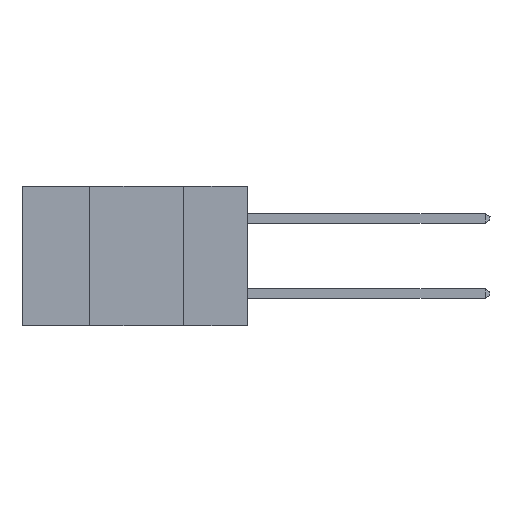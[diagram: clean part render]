
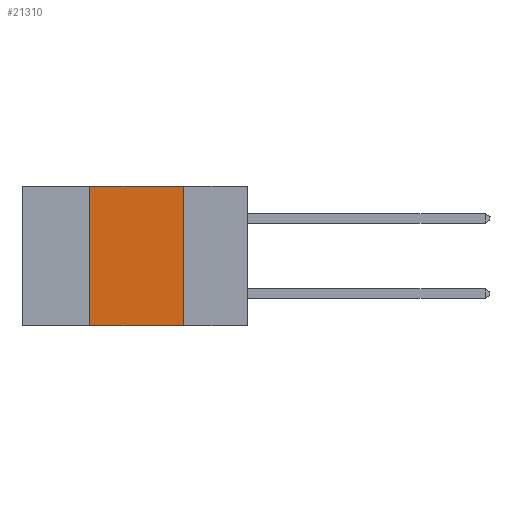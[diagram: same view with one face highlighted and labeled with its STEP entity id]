
A CAD part, left-side view. The second image highlights one B-rep face of the part: STEP entity #21310.
In plain terms, the highlighted planar face has unit normal (-1, 0, 0).
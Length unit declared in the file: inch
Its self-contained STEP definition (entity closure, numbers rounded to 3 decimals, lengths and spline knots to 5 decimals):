
#32 = LINE ( 'NONE', #14050, #11508 ) ;
#1188 = ORIENTED_EDGE ( 'NONE', *, *, #3543, .T. ) ;
#1800 = VERTEX_POINT ( 'NONE', #26650 ) ;
#2411 = FACE_OUTER_BOUND ( 'NONE', #24719, .T. ) ;
#3543 = EDGE_CURVE ( 'NONE', #23350, #1800, #4987, .T. ) ;
#4109 = LINE ( 'NONE', #23231, #20281 ) ;
#4679 = CARTESIAN_POINT ( 'NONE',  ( 0., 0.42, -0.37 ) ) ;
#4723 = EDGE_CURVE ( 'NONE', #13473, #17264, #8897, .T. ) ;
#4987 = LINE ( 'NONE', #22620, #21897 ) ;
#6305 = AXIS2_PLACEMENT_3D ( 'NONE', #25341, #27578, #13982 ) ;
#7141 = DIRECTION ( 'NONE',  ( 0., 0., 1. ) ) ;
#8897 = LINE ( 'NONE', #28176, #14304 ) ;
#9334 = PLANE ( 'NONE',  #6305 ) ;
#11215 = EDGE_CURVE ( 'NONE', #23350, #13473, #4109, .T. ) ;
#11508 = VECTOR ( 'NONE', #25408, 39.37008 ) ;
#11934 = ORIENTED_EDGE ( 'NONE', *, *, #4723, .F. ) ;
#13473 = VERTEX_POINT ( 'NONE', #17204 ) ;
#13982 = DIRECTION ( 'NONE',  ( 0., 0., -1. ) ) ;
#14050 = CARTESIAN_POINT ( 'NONE',  ( 0., 0.17, 0. ) ) ;
#14304 = VECTOR ( 'NONE', #16811, 39.37008 ) ;
#14314 = EDGE_CURVE ( 'NONE', #17264, #1800, #32, .T. ) ;
#16811 = DIRECTION ( 'NONE',  ( 0., -1., 0. ) ) ;
#17204 = CARTESIAN_POINT ( 'NONE',  ( 0., 0.42, 0. ) ) ;
#17264 = VERTEX_POINT ( 'NONE', #27848 ) ;
#18077 = ORIENTED_EDGE ( 'NONE', *, *, #11215, .F. ) ;
#20281 = VECTOR ( 'NONE', #7141, 39.37008 ) ;
#21310 = ADVANCED_FACE ( 'NONE', ( #2411 ), #9334, .F. ) ;
#21897 = VECTOR ( 'NONE', #22156, 39.37008 ) ;
#22156 = DIRECTION ( 'NONE',  ( 0., -1., 0. ) ) ;
#22620 = CARTESIAN_POINT ( 'NONE',  ( 0., 0.6, -0.37 ) ) ;
#23231 = CARTESIAN_POINT ( 'NONE',  ( 0., 0.42, 0. ) ) ;
#23350 = VERTEX_POINT ( 'NONE', #4679 ) ;
#24719 = EDGE_LOOP ( 'NONE', ( #29337, #11934, #18077, #1188 ) ) ;
#25341 = CARTESIAN_POINT ( 'NONE',  ( 0., 0.6, 0. ) ) ;
#25408 = DIRECTION ( 'NONE',  ( 0., 0., -1. ) ) ;
#26650 = CARTESIAN_POINT ( 'NONE',  ( 0., 0.17, -0.37 ) ) ;
#27578 = DIRECTION ( 'NONE',  ( 1., 0., 0. ) ) ;
#27848 = CARTESIAN_POINT ( 'NONE',  ( 0., 0.17, 0. ) ) ;
#28176 = CARTESIAN_POINT ( 'NONE',  ( 0., 0.6, 0. ) ) ;
#29337 = ORIENTED_EDGE ( 'NONE', *, *, #14314, .F. ) ;
